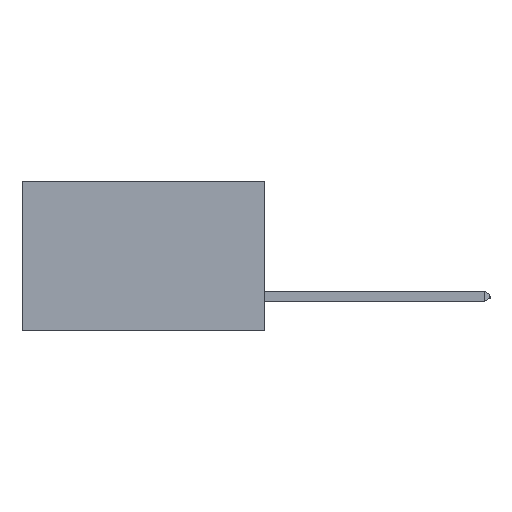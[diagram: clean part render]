
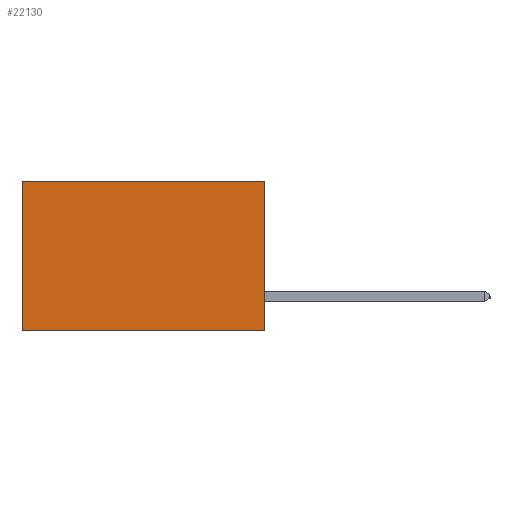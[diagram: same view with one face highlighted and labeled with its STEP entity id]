
A CAD part, left-side view. The second image highlights one B-rep face of the part: STEP entity #22130.
In plain terms, the highlighted planar face has unit normal (-1, 0, 0).
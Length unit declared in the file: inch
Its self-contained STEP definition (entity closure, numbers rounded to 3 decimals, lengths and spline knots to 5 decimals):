
#867 = FACE_OUTER_BOUND ( 'NONE', #21615, .T. ) ;
#1208 = VERTEX_POINT ( 'NONE', #20898 ) ;
#1607 = DIRECTION ( 'NONE',  ( 0., 0., -1. ) ) ;
#2088 = CARTESIAN_POINT ( 'NONE',  ( 0.298, 0., 0. ) ) ;
#3054 = VERTEX_POINT ( 'NONE', #18807 ) ;
#4076 = CARTESIAN_POINT ( 'NONE',  ( 0.298, 0., 0. ) ) ;
#4708 = CARTESIAN_POINT ( 'NONE',  ( 0.298, 0.6, 0. ) ) ;
#4978 = DIRECTION ( 'NONE',  ( 0., 1., 0. ) ) ;
#6768 = DIRECTION ( 'NONE',  ( 0., 0., -1. ) ) ;
#6976 = LINE ( 'NONE', #4708, #11728 ) ;
#9776 = ORIENTED_EDGE ( 'NONE', *, *, #11767, .F. ) ;
#9809 = EDGE_CURVE ( 'NONE', #25369, #23031, #15531, .T. ) ;
#9952 = EDGE_CURVE ( 'NONE', #23031, #3054, #6976, .T. ) ;
#10156 = VECTOR ( 'NONE', #10319, 39.37008 ) ;
#10319 = DIRECTION ( 'NONE',  ( 0., 1., 0. ) ) ;
#11018 = CARTESIAN_POINT ( 'NONE',  ( 0.298, 0., -0.37 ) ) ;
#11715 = LINE ( 'NONE', #11018, #15815 ) ;
#11728 = VECTOR ( 'NONE', #6768, 39.37008 ) ;
#11767 = EDGE_CURVE ( 'NONE', #25369, #1208, #20737, .T. ) ;
#11840 = PLANE ( 'NONE',  #21091 ) ;
#13872 = DIRECTION ( 'NONE',  ( 1., 0., 0. ) ) ;
#14198 = VECTOR ( 'NONE', #20211, 39.37008 ) ;
#14345 = CARTESIAN_POINT ( 'NONE',  ( 0.298, 0.6, 0. ) ) ;
#15531 = LINE ( 'NONE', #2088, #10156 ) ;
#15815 = VECTOR ( 'NONE', #4978, 39.37008 ) ;
#16207 = ORIENTED_EDGE ( 'NONE', *, *, #9809, .T. ) ;
#16218 = CARTESIAN_POINT ( 'NONE',  ( 0.298, 0., 0. ) ) ;
#18807 = CARTESIAN_POINT ( 'NONE',  ( 0.298, 0.6, -0.37 ) ) ;
#18973 = EDGE_CURVE ( 'NONE', #1208, #3054, #11715, .T. ) ;
#20211 = DIRECTION ( 'NONE',  ( 0., 0., -1. ) ) ;
#20737 = LINE ( 'NONE', #4076, #14198 ) ;
#20898 = CARTESIAN_POINT ( 'NONE',  ( 0.298, 0., -0.37 ) ) ;
#21091 = AXIS2_PLACEMENT_3D ( 'NONE', #23745, #13872, #1607 ) ;
#21615 = EDGE_LOOP ( 'NONE', ( #22331, #24457, #9776, #16207 ) ) ;
#22130 = ADVANCED_FACE ( 'NONE', ( #867 ), #11840, .F. ) ;
#22331 = ORIENTED_EDGE ( 'NONE', *, *, #9952, .T. ) ;
#23031 = VERTEX_POINT ( 'NONE', #14345 ) ;
#23745 = CARTESIAN_POINT ( 'NONE',  ( 0.298, 0., 0. ) ) ;
#24457 = ORIENTED_EDGE ( 'NONE', *, *, #18973, .F. ) ;
#25369 = VERTEX_POINT ( 'NONE', #16218 ) ;
